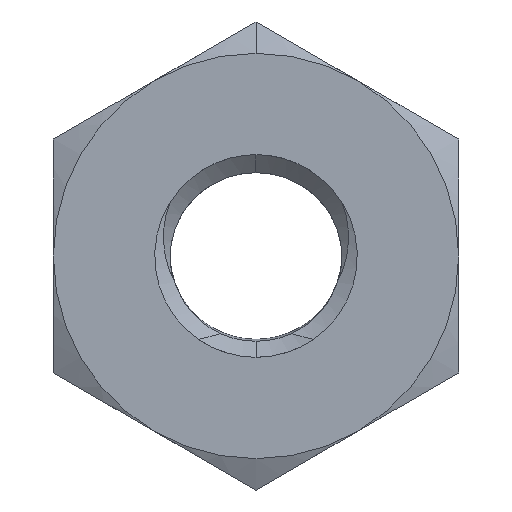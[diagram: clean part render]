
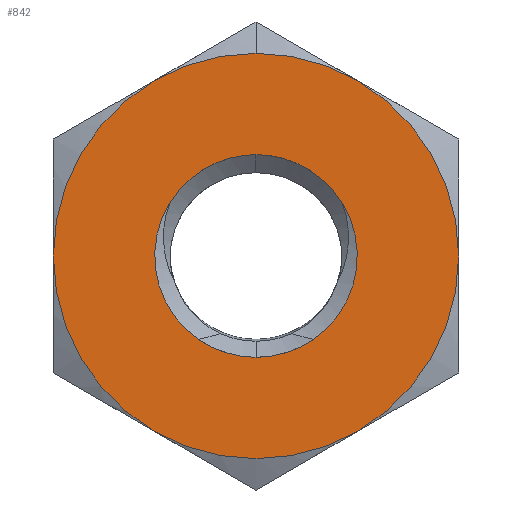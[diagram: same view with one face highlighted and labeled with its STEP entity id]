
A CAD part, front view. The second image highlights one B-rep face of the part: STEP entity #842.
In plain terms, the highlighted planar face has unit normal (0, -1, 0).
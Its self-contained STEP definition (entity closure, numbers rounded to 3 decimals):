
#6 = VERTEX_POINT ( 'NONE', #1353 ) ;
#14 = EDGE_CURVE ( 'NONE', #1131, #1706, #573, .T. ) ;
#23 = VERTEX_POINT ( 'NONE', #988 ) ;
#31 = EDGE_CURVE ( 'NONE', #1959, #1131, #604, .T. ) ;
#36 = CARTESIAN_POINT ( 'NONE',  ( 0., -0.8, 0. ) ) ;
#42 = EDGE_CURVE ( 'NONE', #1228, #1238, #393, .T. ) ;
#46 = EDGE_CURVE ( 'NONE', #23, #941, #878, .T. ) ;
#56 = ORIENTED_EDGE ( 'NONE', *, *, #46, .F. ) ;
#71 = EDGE_CURVE ( 'NONE', #1238, #1612, #202, .T. ) ;
#103 = VERTEX_POINT ( 'NONE', #844 ) ;
#110 = CARTESIAN_POINT ( 'NONE',  ( 0., -0.8, 0. ) ) ;
#115 = ORIENTED_EDGE ( 'NONE', *, *, #453, .T. ) ;
#127 = CARTESIAN_POINT ( 'NONE',  ( -0.067, -0.8, 0.997 ) ) ;
#130 = CARTESIAN_POINT ( 'NONE',  ( 0., -0.8, 0. ) ) ;
#134 = ORIENTED_EDGE ( 'NONE', *, *, #234, .T. ) ;
#186 = DIRECTION ( 'NONE',  ( 0., 0., -1. ) ) ;
#202 = CIRCLE ( 'NONE', #1016, 2. ) ;
#234 = EDGE_CURVE ( 'NONE', #1006, #1031, #1617, .T. ) ;
#243 = EDGE_CURVE ( 'NONE', #1031, #1228, #1722, .T. ) ;
#271 = AXIS2_PLACEMENT_3D ( 'NONE', #1018, #921, #1915 ) ;
#276 = CIRCLE ( 'NONE', #1941, 1. ) ;
#288 = PLANE ( 'NONE',  #1452 ) ;
#291 = DIRECTION ( 'NONE',  ( 0., 0., -1. ) ) ;
#340 = AXIS2_PLACEMENT_3D ( 'NONE', #761, #1834, #929 ) ;
#343 = CARTESIAN_POINT ( 'NONE',  ( 1., -0.8, 1.732 ) ) ;
#362 = CIRCLE ( 'NONE', #1701, 2. ) ;
#372 = ORIENTED_EDGE ( 'NONE', *, *, #415, .F. ) ;
#393 = CIRCLE ( 'NONE', #607, 2. ) ;
#414 = CARTESIAN_POINT ( 'NONE',  ( 0., -0.8, 0. ) ) ;
#415 = EDGE_CURVE ( 'NONE', #1706, #463, #882, .T. ) ;
#453 = EDGE_CURVE ( 'NONE', #777, #1006, #860, .T. ) ;
#463 = VERTEX_POINT ( 'NONE', #1682 ) ;
#471 = CARTESIAN_POINT ( 'NONE',  ( -0.101, -0.8, 0.995 ) ) ;
#511 = AXIS2_PLACEMENT_3D ( 'NONE', #1994, #778, #1671 ) ;
#519 = DIRECTION ( 'NONE',  ( 0., -1., 0. ) ) ;
#532 = CARTESIAN_POINT ( 'NONE',  ( 0.566, -0.8, -0.824 ) ) ;
#533 = ORIENTED_EDGE ( 'NONE', *, *, #561, .T. ) ;
#556 = DIRECTION ( 'NONE',  ( 0., -1., 0. ) ) ;
#561 = EDGE_CURVE ( 'NONE', #1612, #6, #362, .T. ) ;
#567 = CARTESIAN_POINT ( 'NONE',  ( -0.566, -0.8, -0.824 ) ) ;
#573 = CIRCLE ( 'NONE', #271, 1. ) ;
#590 = DIRECTION ( 'NONE',  ( 0., 0., -1. ) ) ;
#602 = DIRECTION ( 'NONE',  ( 0., -1., 0. ) ) ;
#604 = CIRCLE ( 'NONE', #511, 1. ) ;
#607 = AXIS2_PLACEMENT_3D ( 'NONE', #1549, #1718, #1628 ) ;
#713 = FACE_OUTER_BOUND ( 'NONE', #1939, .T. ) ;
#732 = DIRECTION ( 'NONE',  ( 0., -1., 0. ) ) ;
#753 = EDGE_CURVE ( 'NONE', #103, #23, #276, .T. ) ;
#761 = CARTESIAN_POINT ( 'NONE',  ( 0., -0.8, 0. ) ) ;
#764 = CARTESIAN_POINT ( 'NONE',  ( 0., -0.8, 0. ) ) ;
#777 = VERTEX_POINT ( 'NONE', #1229 ) ;
#778 = DIRECTION ( 'NONE',  ( 0., -1., 0. ) ) ;
#779 = DIRECTION ( 'NONE',  ( 0., 0., -1. ) ) ;
#782 = CARTESIAN_POINT ( 'NONE',  ( -1., -0.8, -1.732 ) ) ;
#842 = ADVANCED_FACE ( 'NONE', ( #713, #1188 ), #288, .T. ) ;
#844 = CARTESIAN_POINT ( 'NONE',  ( 0.848, -0.8, 0.53 ) ) ;
#852 = CARTESIAN_POINT ( 'NONE',  ( 0., -0.8, 0.999 ) ) ;
#855 = EDGE_LOOP ( 'NONE', ( #1426, #1325, #372, #1731, #900, #1094, #56, #1190 ) ) ;
#860 = CIRCLE ( 'NONE', #1668, 2. ) ;
#878 = B_SPLINE_CURVE_WITH_KNOTS ( 'NONE', 3,
 ( #1960, #1966, #1215, #852 ),
 .UNSPECIFIED., .F., .F.,
 ( 4, 4 ),
 ( 0., 0.5 ),
 .UNSPECIFIED. ) ;
#882 = CIRCLE ( 'NONE', #1432, 1. ) ;
#896 = ORIENTED_EDGE ( 'NONE', *, *, #42, .T. ) ;
#900 = ORIENTED_EDGE ( 'NONE', *, *, #31, .F. ) ;
#906 = DIRECTION ( 'NONE',  ( 0., 0., -1. ) ) ;
#921 = DIRECTION ( 'NONE',  ( 0., -1., 0. ) ) ;
#929 = DIRECTION ( 'NONE',  ( 0., 0., -1. ) ) ;
#941 = VERTEX_POINT ( 'NONE', #1408 ) ;
#988 = CARTESIAN_POINT ( 'NONE',  ( 0.101, -0.8, 0.995 ) ) ;
#995 = AXIS2_PLACEMENT_3D ( 'NONE', #1651, #732, #1808 ) ;
#998 = EDGE_CURVE ( 'NONE', #1885, #103, #1284, .T. ) ;
#1006 = VERTEX_POINT ( 'NONE', #1688 ) ;
#1016 = AXIS2_PLACEMENT_3D ( 'NONE', #110, #1306, #1650 ) ;
#1018 = CARTESIAN_POINT ( 'NONE',  ( 0., -0.8, 0. ) ) ;
#1031 = VERTEX_POINT ( 'NONE', #782 ) ;
#1069 = AXIS2_PLACEMENT_3D ( 'NONE', #36, #1148, #186 ) ;
#1081 = CARTESIAN_POINT ( 'NONE',  ( 1., -0.8, -1.732 ) ) ;
#1088 = CARTESIAN_POINT ( 'NONE',  ( 2., -0.8, -1.155 ) ) ;
#1094 = ORIENTED_EDGE ( 'NONE', *, *, #1240, .F. ) ;
#1098 = AXIS2_PLACEMENT_3D ( 'NONE', #1435, #519, #1588 ) ;
#1131 = VERTEX_POINT ( 'NONE', #1344 ) ;
#1139 = EDGE_CURVE ( 'NONE', #6, #777, #1519, .T. ) ;
#1148 = DIRECTION ( 'NONE',  ( 0., -1., 0. ) ) ;
#1153 = ORIENTED_EDGE ( 'NONE', *, *, #1139, .T. ) ;
#1158 = AXIS2_PLACEMENT_3D ( 'NONE', #130, #1242, #291 ) ;
#1188 = FACE_BOUND ( 'NONE', #855, .T. ) ;
#1190 = ORIENTED_EDGE ( 'NONE', *, *, #753, .F. ) ;
#1215 = CARTESIAN_POINT ( 'NONE',  ( 0.034, -0.8, 0.999 ) ) ;
#1228 = VERTEX_POINT ( 'NONE', #1081 ) ;
#1229 = CARTESIAN_POINT ( 'NONE',  ( -1., -0.8, 1.732 ) ) ;
#1236 = CARTESIAN_POINT ( 'NONE',  ( -0.101, -0.8, 0.995 ) ) ;
#1238 = VERTEX_POINT ( 'NONE', #1974 ) ;
#1240 = EDGE_CURVE ( 'NONE', #941, #1959, #1301, .T. ) ;
#1242 = DIRECTION ( 'NONE',  ( 0., -1., 0. ) ) ;
#1284 = CIRCLE ( 'NONE', #340, 1. ) ;
#1301 = B_SPLINE_CURVE_WITH_KNOTS ( 'NONE', 3,
 ( #1981, #1831, #127, #1236 ),
 .UNSPECIFIED., .F., .F.,
 ( 4, 4 ),
 ( 0.5, 1. ),
 .UNSPECIFIED. ) ;
#1306 = DIRECTION ( 'NONE',  ( 0., -1., 0. ) ) ;
#1325 = ORIENTED_EDGE ( 'NONE', *, *, #1465, .F. ) ;
#1344 = CARTESIAN_POINT ( 'NONE',  ( -0.848, -0.8, 0.53 ) ) ;
#1353 = CARTESIAN_POINT ( 'NONE',  ( 0., -0.8, 2. ) ) ;
#1408 = CARTESIAN_POINT ( 'NONE',  ( 0., -0.8, 0.999 ) ) ;
#1426 = ORIENTED_EDGE ( 'NONE', *, *, #998, .F. ) ;
#1432 = AXIS2_PLACEMENT_3D ( 'NONE', #1510, #602, #1672 ) ;
#1435 = CARTESIAN_POINT ( 'NONE',  ( 0., -0.8, 0. ) ) ;
#1452 = AXIS2_PLACEMENT_3D ( 'NONE', #1088, #1693, #779 ) ;
#1465 = EDGE_CURVE ( 'NONE', #463, #1885, #1740, .T. ) ;
#1471 = CARTESIAN_POINT ( 'NONE',  ( 0., -0.8, 0. ) ) ;
#1499 = DIRECTION ( 'NONE',  ( 0., -1., 0. ) ) ;
#1510 = CARTESIAN_POINT ( 'NONE',  ( 0., -0.8, 0. ) ) ;
#1519 = CIRCLE ( 'NONE', #995, 2. ) ;
#1549 = CARTESIAN_POINT ( 'NONE',  ( 0., -0.8, 0. ) ) ;
#1574 = ORIENTED_EDGE ( 'NONE', *, *, #71, .T. ) ;
#1588 = DIRECTION ( 'NONE',  ( 0., 0., -1. ) ) ;
#1612 = VERTEX_POINT ( 'NONE', #343 ) ;
#1617 = CIRCLE ( 'NONE', #1069, 2. ) ;
#1628 = DIRECTION ( 'NONE',  ( 0., 0., -1. ) ) ;
#1631 = DIRECTION ( 'NONE',  ( 0., 0., -1. ) ) ;
#1650 = DIRECTION ( 'NONE',  ( 0., 0., -1. ) ) ;
#1651 = CARTESIAN_POINT ( 'NONE',  ( 0., -0.8, 0. ) ) ;
#1668 = AXIS2_PLACEMENT_3D ( 'NONE', #764, #1835, #906 ) ;
#1671 = DIRECTION ( 'NONE',  ( 0., 0., -1. ) ) ;
#1672 = DIRECTION ( 'NONE',  ( 0., 0., -1. ) ) ;
#1682 = CARTESIAN_POINT ( 'NONE',  ( 0., -0.8, -1. ) ) ;
#1688 = CARTESIAN_POINT ( 'NONE',  ( -2., -0.8, 0. ) ) ;
#1693 = DIRECTION ( 'NONE',  ( 0., -1., 0. ) ) ;
#1701 = AXIS2_PLACEMENT_3D ( 'NONE', #414, #1499, #590 ) ;
#1706 = VERTEX_POINT ( 'NONE', #567 ) ;
#1718 = DIRECTION ( 'NONE',  ( 0., -1., 0. ) ) ;
#1722 = CIRCLE ( 'NONE', #1098, 2. ) ;
#1731 = ORIENTED_EDGE ( 'NONE', *, *, #14, .F. ) ;
#1740 = CIRCLE ( 'NONE', #1158, 1. ) ;
#1803 = ORIENTED_EDGE ( 'NONE', *, *, #243, .T. ) ;
#1808 = DIRECTION ( 'NONE',  ( 0., 0., -1. ) ) ;
#1831 = CARTESIAN_POINT ( 'NONE',  ( -0.034, -0.8, 0.999 ) ) ;
#1834 = DIRECTION ( 'NONE',  ( 0., -1., 0. ) ) ;
#1835 = DIRECTION ( 'NONE',  ( 0., -1., 0. ) ) ;
#1885 = VERTEX_POINT ( 'NONE', #532 ) ;
#1915 = DIRECTION ( 'NONE',  ( 0., 0., -1. ) ) ;
#1939 = EDGE_LOOP ( 'NONE', ( #134, #1803, #896, #1574, #533, #1153, #115 ) ) ;
#1941 = AXIS2_PLACEMENT_3D ( 'NONE', #1471, #556, #1631 ) ;
#1959 = VERTEX_POINT ( 'NONE', #471 ) ;
#1960 = CARTESIAN_POINT ( 'NONE',  ( 0.101, -0.8, 0.995 ) ) ;
#1966 = CARTESIAN_POINT ( 'NONE',  ( 0.067, -0.8, 0.997 ) ) ;
#1974 = CARTESIAN_POINT ( 'NONE',  ( 2., -0.8, 0. ) ) ;
#1981 = CARTESIAN_POINT ( 'NONE',  ( 0., -0.8, 0.999 ) ) ;
#1994 = CARTESIAN_POINT ( 'NONE',  ( 0., -0.8, 0. ) ) ;
